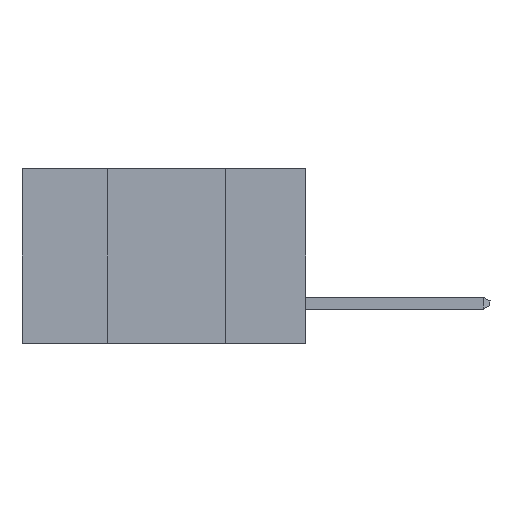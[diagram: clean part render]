
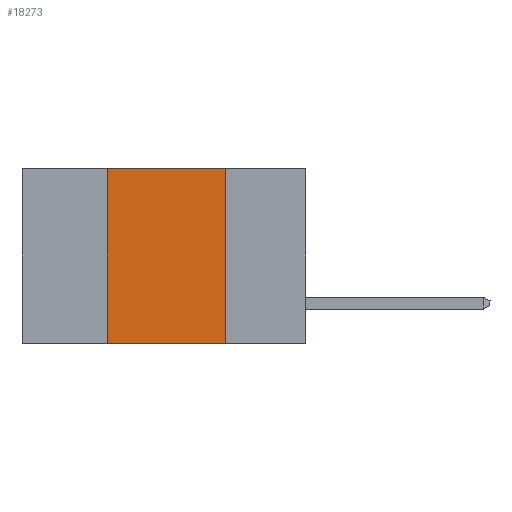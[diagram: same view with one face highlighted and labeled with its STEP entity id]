
A CAD part, left-side view. The second image highlights one B-rep face of the part: STEP entity #18273.
In plain terms, the highlighted planar face has unit normal (-1, 0, 0).
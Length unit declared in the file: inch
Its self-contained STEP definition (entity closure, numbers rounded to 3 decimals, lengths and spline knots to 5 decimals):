
#954 = PLANE ( 'NONE',  #12567 ) ;
#1150 = DIRECTION ( 'NONE',  ( 0., 0., -1. ) ) ;
#1441 = VECTOR ( 'NONE', #11286, 39.37008 ) ;
#1963 = EDGE_CURVE ( 'NONE', #6074, #15661, #16835, .T. ) ;
#2937 = CARTESIAN_POINT ( 'NONE',  ( 0., 0.42, -0.37 ) ) ;
#5103 = VERTEX_POINT ( 'NONE', #15408 ) ;
#5257 = DIRECTION ( 'NONE',  ( 0., -1., 0. ) ) ;
#5265 = ORIENTED_EDGE ( 'NONE', *, *, #8927, .T. ) ;
#6074 = VERTEX_POINT ( 'NONE', #19878 ) ;
#6112 = VECTOR ( 'NONE', #14360, 39.37008 ) ;
#6446 = LINE ( 'NONE', #16972, #6112 ) ;
#8771 = CARTESIAN_POINT ( 'NONE',  ( 0., 0.6, 0. ) ) ;
#8927 = EDGE_CURVE ( 'NONE', #6074, #11640, #14896, .T. ) ;
#8944 = ORIENTED_EDGE ( 'NONE', *, *, #8962, .F. ) ;
#8962 = EDGE_CURVE ( 'NONE', #5103, #11640, #13284, .T. ) ;
#11072 = EDGE_CURVE ( 'NONE', #15661, #5103, #6446, .T. ) ;
#11286 = DIRECTION ( 'NONE',  ( 0., 0., 1. ) ) ;
#11509 = ORIENTED_EDGE ( 'NONE', *, *, #11072, .F. ) ;
#11640 = VERTEX_POINT ( 'NONE', #16126 ) ;
#12567 = AXIS2_PLACEMENT_3D ( 'NONE', #8771, #14960, #1150 ) ;
#13284 = LINE ( 'NONE', #18016, #14324 ) ;
#14324 = VECTOR ( 'NONE', #16404, 39.37008 ) ;
#14360 = DIRECTION ( 'NONE',  ( 0., -1., 0. ) ) ;
#14896 = LINE ( 'NONE', #17912, #16575 ) ;
#14960 = DIRECTION ( 'NONE',  ( 1., 0., 0. ) ) ;
#15408 = CARTESIAN_POINT ( 'NONE',  ( 0., 0.17, 0. ) ) ;
#15661 = VERTEX_POINT ( 'NONE', #19723 ) ;
#16126 = CARTESIAN_POINT ( 'NONE',  ( 0., 0.17, -0.37 ) ) ;
#16404 = DIRECTION ( 'NONE',  ( 0., 0., -1. ) ) ;
#16469 = FACE_OUTER_BOUND ( 'NONE', #16578, .T. ) ;
#16575 = VECTOR ( 'NONE', #5257, 39.37008 ) ;
#16578 = EDGE_LOOP ( 'NONE', ( #8944, #11509, #19886, #5265 ) ) ;
#16835 = LINE ( 'NONE', #2937, #1441 ) ;
#16972 = CARTESIAN_POINT ( 'NONE',  ( 0., 0.6, 0. ) ) ;
#17912 = CARTESIAN_POINT ( 'NONE',  ( 0., 0.6, -0.37 ) ) ;
#18016 = CARTESIAN_POINT ( 'NONE',  ( 0., 0.17, -0.37 ) ) ;
#18273 = ADVANCED_FACE ( 'NONE', ( #16469 ), #954, .F. ) ;
#19723 = CARTESIAN_POINT ( 'NONE',  ( 0., 0.42, 0. ) ) ;
#19878 = CARTESIAN_POINT ( 'NONE',  ( 0., 0.42, -0.37 ) ) ;
#19886 = ORIENTED_EDGE ( 'NONE', *, *, #1963, .F. ) ;
